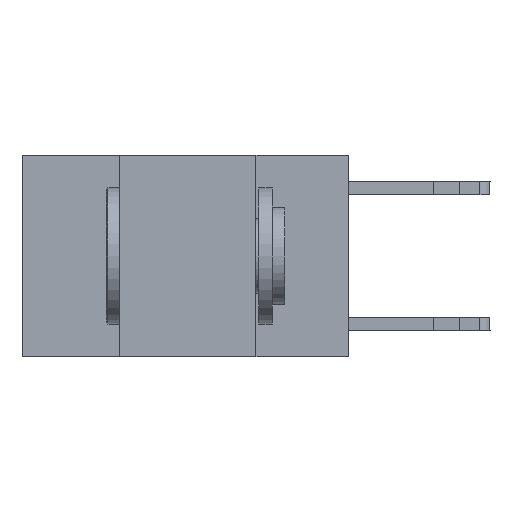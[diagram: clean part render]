
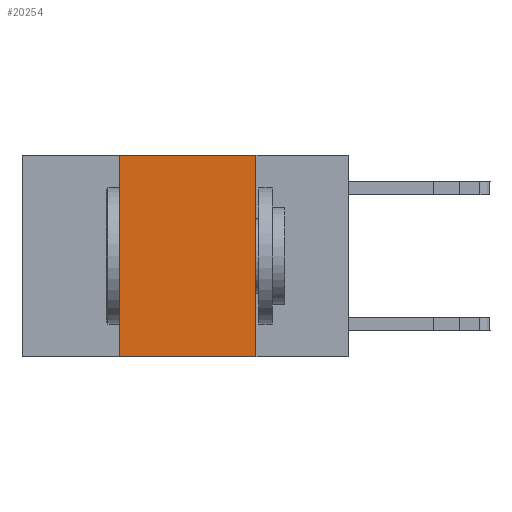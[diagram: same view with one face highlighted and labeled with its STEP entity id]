
A CAD part, left-side view. The second image highlights one B-rep face of the part: STEP entity #20254.
In plain terms, the highlighted planar face has unit normal (-1, 0, 0).
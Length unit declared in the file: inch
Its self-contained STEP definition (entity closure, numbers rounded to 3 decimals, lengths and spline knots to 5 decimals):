
#655 = VERTEX_POINT ( 'NONE', #7344 ) ;
#695 = ORIENTED_EDGE ( 'NONE', *, *, #4918, .T. ) ;
#878 = VECTOR ( 'NONE', #18329, 39.37008 ) ;
#1033 = CARTESIAN_POINT ( 'NONE',  ( 0., 0.6, 0. ) ) ;
#1835 = VERTEX_POINT ( 'NONE', #7856 ) ;
#3117 = EDGE_CURVE ( 'NONE', #655, #15601, #4526, .T. ) ;
#4281 = DIRECTION ( 'NONE',  ( 0., -1., 0. ) ) ;
#4526 = LINE ( 'NONE', #4652, #17466 ) ;
#4652 = CARTESIAN_POINT ( 'NONE',  ( 0., 0.17, 0. ) ) ;
#4918 = EDGE_CURVE ( 'NONE', #1835, #15601, #20144, .T. ) ;
#5825 = DIRECTION ( 'NONE',  ( 0., 0., 1. ) ) ;
#6433 = ORIENTED_EDGE ( 'NONE', *, *, #15412, .F. ) ;
#7344 = CARTESIAN_POINT ( 'NONE',  ( 0., 0.17, 0. ) ) ;
#7856 = CARTESIAN_POINT ( 'NONE',  ( 0., 0.42, -0.37 ) ) ;
#8098 = DIRECTION ( 'NONE',  ( 0., 0., -1. ) ) ;
#8605 = AXIS2_PLACEMENT_3D ( 'NONE', #1033, #20256, #8098 ) ;
#8819 = ORIENTED_EDGE ( 'NONE', *, *, #3117, .F. ) ;
#9236 = ORIENTED_EDGE ( 'NONE', *, *, #22817, .F. ) ;
#9257 = CARTESIAN_POINT ( 'NONE',  ( 0., 0.42, 0. ) ) ;
#14417 = LINE ( 'NONE', #19608, #878 ) ;
#14640 = CARTESIAN_POINT ( 'NONE',  ( 0., 0.42, 0. ) ) ;
#15412 = EDGE_CURVE ( 'NONE', #1835, #18707, #21459, .T. ) ;
#15601 = VERTEX_POINT ( 'NONE', #20861 ) ;
#17002 = FACE_OUTER_BOUND ( 'NONE', #18815, .T. ) ;
#17466 = VECTOR ( 'NONE', #22016, 39.37008 ) ;
#17505 = VECTOR ( 'NONE', #5825, 39.37008 ) ;
#18293 = CARTESIAN_POINT ( 'NONE',  ( 0., 0.6, -0.37 ) ) ;
#18329 = DIRECTION ( 'NONE',  ( 0., -1., 0. ) ) ;
#18707 = VERTEX_POINT ( 'NONE', #9257 ) ;
#18815 = EDGE_LOOP ( 'NONE', ( #8819, #9236, #6433, #695 ) ) ;
#19097 = VECTOR ( 'NONE', #4281, 39.37008 ) ;
#19608 = CARTESIAN_POINT ( 'NONE',  ( 0., 0.6, 0. ) ) ;
#20144 = LINE ( 'NONE', #18293, #19097 ) ;
#20254 = ADVANCED_FACE ( 'NONE', ( #17002 ), #22106, .F. ) ;
#20256 = DIRECTION ( 'NONE',  ( 1., 0., 0. ) ) ;
#20861 = CARTESIAN_POINT ( 'NONE',  ( 0., 0.17, -0.37 ) ) ;
#21459 = LINE ( 'NONE', #14640, #17505 ) ;
#22016 = DIRECTION ( 'NONE',  ( 0., 0., -1. ) ) ;
#22106 = PLANE ( 'NONE',  #8605 ) ;
#22817 = EDGE_CURVE ( 'NONE', #18707, #655, #14417, .T. ) ;
